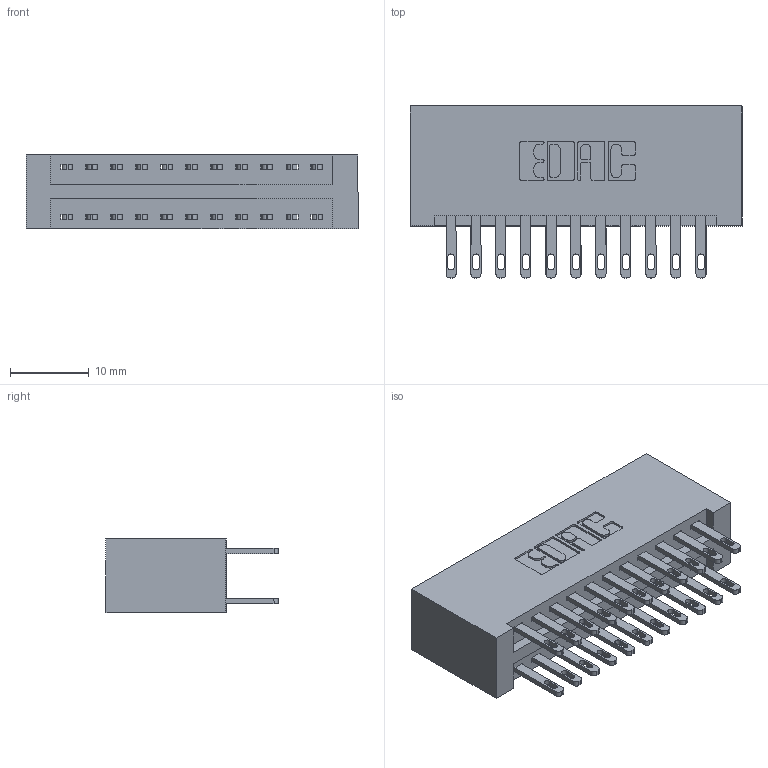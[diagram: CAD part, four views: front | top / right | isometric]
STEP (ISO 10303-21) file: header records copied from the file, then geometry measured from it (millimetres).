
FILE_DESCRIPTION (( 'STEP AP203' ), '1' );
FILE_NAME ('896-022-500-201.STEP', '2021-07-27T16:52:50', ( '' ), ( '' ), 'SwSTEP 2.0', 'SolidWorks 2020', '' );
FILE_SCHEMA (( 'CONFIG_CONTROL_DESIGN' ));
Length unit declared in the file: inch
Products named in the file (3): 896-022-500-201; 345-292-001_345-293-100; 846 Part_No Mounting Lugs
Assembly tree (23 placements, depth 2):
  896-022-500-201
    846 Part_No Mounting Lugs
    345-292-001_345-293-100  x22
Bounding box: 42.16 x 21.84 x 9.4 mm (x, y, z)
Volume: 4511.3 mm3; surface area: 6107.2 mm2
Topology: 23 solids, 23 shells, 1170 faces, 3539 edges, 2358 vertices
Faces by surface type: plane 710, cylinder 460
Entity records: 11005 total; most frequent: CARTESIAN_POINT 1852, ORIENTED_EDGE 1786, DIRECTION 1681, EDGE_CURVE 893, LINE 721, VECTOR 721, VERTEX_POINT 594, AXIS2_PLACEMENT_3D 480
